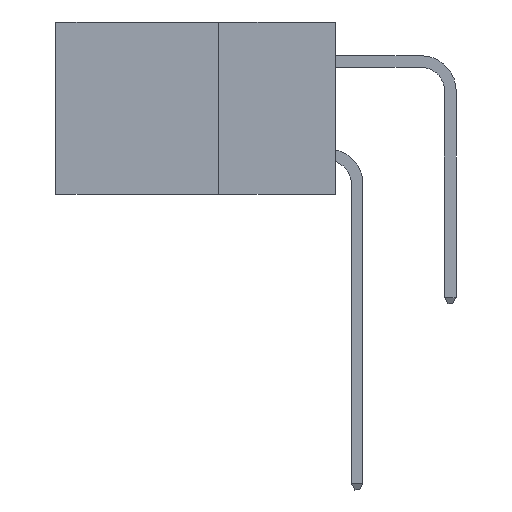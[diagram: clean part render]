
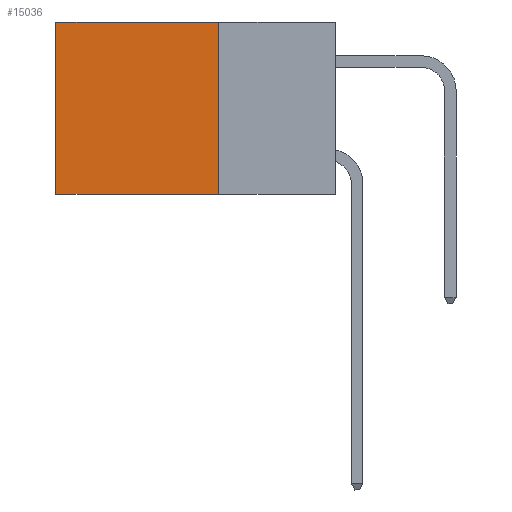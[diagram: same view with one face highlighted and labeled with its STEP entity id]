
A CAD part, left-side view. The second image highlights one B-rep face of the part: STEP entity #15036.
In plain terms, the highlighted planar face has unit normal (-1, 0, 0).
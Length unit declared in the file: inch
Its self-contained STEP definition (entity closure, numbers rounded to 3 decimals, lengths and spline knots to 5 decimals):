
#945 = ORIENTED_EDGE ( 'NONE', *, *, #6600, .T. ) ;
#1262 = ORIENTED_EDGE ( 'NONE', *, *, #12617, .F. ) ;
#1757 = CARTESIAN_POINT ( 'NONE',  ( 0.2875, 0.6, -0.37 ) ) ;
#1981 = VECTOR ( 'NONE', #15993, 39.37008 ) ;
#2183 = CARTESIAN_POINT ( 'NONE',  ( 0.2875, 0.25, -0.37 ) ) ;
#2763 = EDGE_CURVE ( 'NONE', #5114, #17970, #5618, .T. ) ;
#2782 = CARTESIAN_POINT ( 'NONE',  ( 0.2875, 0.6, 0. ) ) ;
#3082 = LINE ( 'NONE', #11748, #11414 ) ;
#3382 = EDGE_CURVE ( 'NONE', #5114, #11624, #3082, .T. ) ;
#3445 = AXIS2_PLACEMENT_3D ( 'NONE', #14621, #17692, #8508 ) ;
#4986 = EDGE_LOOP ( 'NONE', ( #945, #1262, #15990, #17367 ) ) ;
#5114 = VERTEX_POINT ( 'NONE', #6746 ) ;
#5192 = FACE_OUTER_BOUND ( 'NONE', #4986, .T. ) ;
#5225 = CARTESIAN_POINT ( 'NONE',  ( 0.2875, 0.25, -0.37 ) ) ;
#5618 = LINE ( 'NONE', #14722, #13369 ) ;
#6600 = EDGE_CURVE ( 'NONE', #11624, #7008, #18729, .T. ) ;
#6746 = CARTESIAN_POINT ( 'NONE',  ( 0.2875, 0.25, 0. ) ) ;
#7008 = VERTEX_POINT ( 'NONE', #1757 ) ;
#8508 = DIRECTION ( 'NONE',  ( 0., 0., -1. ) ) ;
#11414 = VECTOR ( 'NONE', #16295, 39.37008 ) ;
#11624 = VERTEX_POINT ( 'NONE', #2782 ) ;
#11748 = CARTESIAN_POINT ( 'NONE',  ( 0.2875, 0.25, 0. ) ) ;
#12617 = EDGE_CURVE ( 'NONE', #17970, #7008, #17044, .T. ) ;
#13369 = VECTOR ( 'NONE', #17793, 39.37008 ) ;
#14555 = PLANE ( 'NONE',  #3445 ) ;
#14621 = CARTESIAN_POINT ( 'NONE',  ( 0.2875, 0.25, 0. ) ) ;
#14722 = CARTESIAN_POINT ( 'NONE',  ( 0.2875, 0.25, 0. ) ) ;
#15036 = ADVANCED_FACE ( 'NONE', ( #5192 ), #14555, .F. ) ;
#15990 = ORIENTED_EDGE ( 'NONE', *, *, #2763, .F. ) ;
#15993 = DIRECTION ( 'NONE',  ( 0., 1., 0. ) ) ;
#16295 = DIRECTION ( 'NONE',  ( 0., 1., 0. ) ) ;
#16396 = DIRECTION ( 'NONE',  ( 0., 0., -1. ) ) ;
#17044 = LINE ( 'NONE', #5225, #1981 ) ;
#17367 = ORIENTED_EDGE ( 'NONE', *, *, #3382, .T. ) ;
#17692 = DIRECTION ( 'NONE',  ( 1., 0., 0. ) ) ;
#17793 = DIRECTION ( 'NONE',  ( 0., 0., -1. ) ) ;
#17970 = VERTEX_POINT ( 'NONE', #2183 ) ;
#18246 = VECTOR ( 'NONE', #16396, 39.37008 ) ;
#18729 = LINE ( 'NONE', #19407, #18246 ) ;
#19407 = CARTESIAN_POINT ( 'NONE',  ( 0.2875, 0.6, 0. ) ) ;
